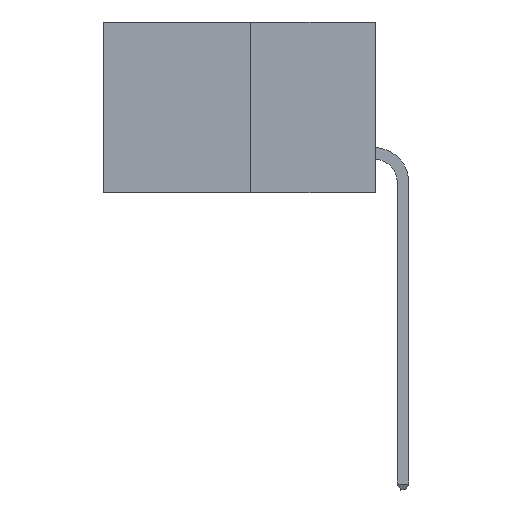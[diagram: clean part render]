
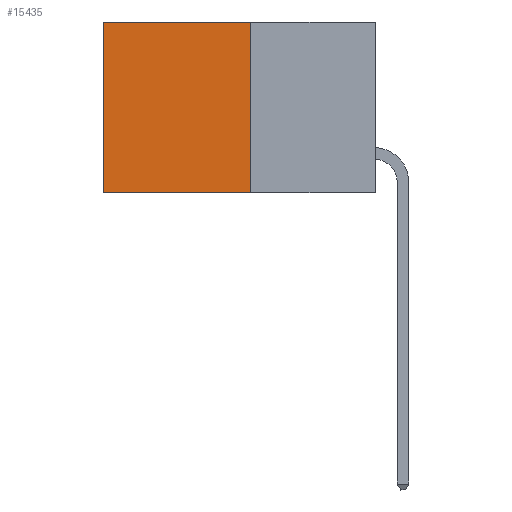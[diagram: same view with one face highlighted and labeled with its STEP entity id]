
A CAD part, left-side view. The second image highlights one B-rep face of the part: STEP entity #15435.
In plain terms, the highlighted planar face has unit normal (-1, 0, 0).
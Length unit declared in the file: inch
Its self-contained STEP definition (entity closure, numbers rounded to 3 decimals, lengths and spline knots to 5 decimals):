
#160 = CARTESIAN_POINT ( 'NONE',  ( 0.277, 0.59, -0.37 ) ) ;
#468 = ORIENTED_EDGE ( 'NONE', *, *, #12056, .T. ) ;
#1672 = LINE ( 'NONE', #6594, #15317 ) ;
#2845 = ORIENTED_EDGE ( 'NONE', *, *, #11724, .F. ) ;
#3216 = VECTOR ( 'NONE', #4340, 39.37008 ) ;
#4340 = DIRECTION ( 'NONE',  ( 0., 1., 0. ) ) ;
#4840 = EDGE_CURVE ( 'NONE', #12134, #8371, #16706, .T. ) ;
#6594 = CARTESIAN_POINT ( 'NONE',  ( 0.277, 0.27, 0. ) ) ;
#6669 = EDGE_CURVE ( 'NONE', #6780, #8420, #12108, .T. ) ;
#6780 = VERTEX_POINT ( 'NONE', #8664 ) ;
#6921 = LINE ( 'NONE', #11178, #3216 ) ;
#8018 = CARTESIAN_POINT ( 'NONE',  ( 0.277, 0.27, -0.37 ) ) ;
#8371 = VERTEX_POINT ( 'NONE', #9618 ) ;
#8420 = VERTEX_POINT ( 'NONE', #8018 ) ;
#8664 = CARTESIAN_POINT ( 'NONE',  ( 0.277, 0.27, 0. ) ) ;
#8756 = DIRECTION ( 'NONE',  ( 0., 0., -1. ) ) ;
#9618 = CARTESIAN_POINT ( 'NONE',  ( 0.277, 0.59, -0.37 ) ) ;
#9626 = VECTOR ( 'NONE', #13840, 39.37008 ) ;
#9850 = CARTESIAN_POINT ( 'NONE',  ( 0.277, 0.27, -0.37 ) ) ;
#9892 = DIRECTION ( 'NONE',  ( 0., 0., -1. ) ) ;
#10585 = ORIENTED_EDGE ( 'NONE', *, *, #6669, .F. ) ;
#10929 = CARTESIAN_POINT ( 'NONE',  ( 0.277, 0.59, 0. ) ) ;
#11178 = CARTESIAN_POINT ( 'NONE',  ( 0.277, 0.27, -0.37 ) ) ;
#11724 = EDGE_CURVE ( 'NONE', #8420, #8371, #6921, .T. ) ;
#12056 = EDGE_CURVE ( 'NONE', #6780, #12134, #1672, .T. ) ;
#12108 = LINE ( 'NONE', #9850, #12512 ) ;
#12134 = VERTEX_POINT ( 'NONE', #10929 ) ;
#12512 = VECTOR ( 'NONE', #9892, 39.37008 ) ;
#12883 = ORIENTED_EDGE ( 'NONE', *, *, #4840, .T. ) ;
#13840 = DIRECTION ( 'NONE',  ( 0., 0., -1. ) ) ;
#14081 = PLANE ( 'NONE',  #14220 ) ;
#14220 = AXIS2_PLACEMENT_3D ( 'NONE', #15409, #16726, #8756 ) ;
#14306 = EDGE_LOOP ( 'NONE', ( #12883, #2845, #10585, #468 ) ) ;
#15317 = VECTOR ( 'NONE', #17357, 39.37008 ) ;
#15409 = CARTESIAN_POINT ( 'NONE',  ( 0.277, 0.27, -0.37 ) ) ;
#15435 = ADVANCED_FACE ( 'NONE', ( #15979 ), #14081, .F. ) ;
#15979 = FACE_OUTER_BOUND ( 'NONE', #14306, .T. ) ;
#16706 = LINE ( 'NONE', #160, #9626 ) ;
#16726 = DIRECTION ( 'NONE',  ( 1., 0., 0. ) ) ;
#17357 = DIRECTION ( 'NONE',  ( 0., 1., 0. ) ) ;
